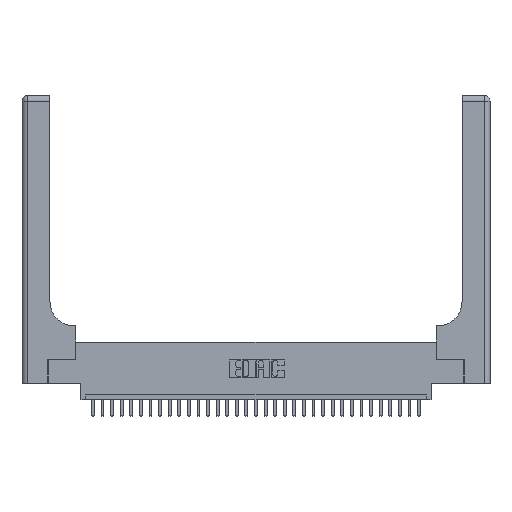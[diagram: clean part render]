
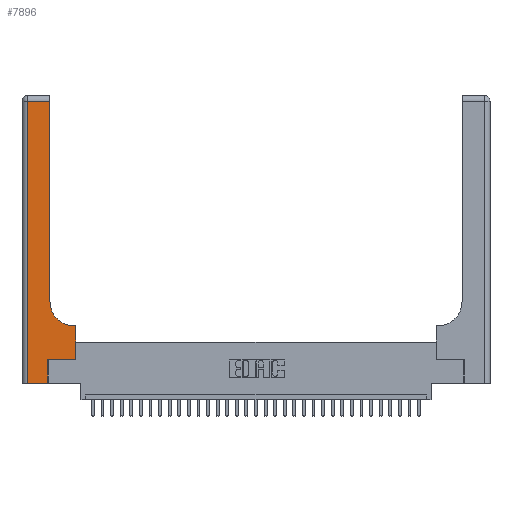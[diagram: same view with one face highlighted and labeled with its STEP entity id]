
A CAD part, top view. The second image highlights one B-rep face of the part: STEP entity #7896.
In plain terms, the highlighted planar face has unit normal (0, 0, 1).
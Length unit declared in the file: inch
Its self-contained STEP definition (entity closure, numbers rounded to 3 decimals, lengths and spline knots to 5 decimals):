
#596 = ORIENTED_EDGE ( 'NONE', *, *, #30596, .T. ) ;
#619 = LINE ( 'NONE', #20753, #26712 ) ;
#670 = VECTOR ( 'NONE', #19049, 39.37008 ) ;
#977 = ORIENTED_EDGE ( 'NONE', *, *, #3471, .T. ) ;
#1004 = VECTOR ( 'NONE', #30805, 39.37008 ) ;
#1244 = CARTESIAN_POINT ( 'NONE',  ( 0.5585, 0.25, 0.37 ) ) ;
#1308 = ORIENTED_EDGE ( 'NONE', *, *, #28252, .T. ) ;
#1707 = CARTESIAN_POINT ( 'NONE',  ( 0.2915, 2.94, 0.37 ) ) ;
#2346 = CARTESIAN_POINT ( 'NONE',  ( 0.5585, 0.6, 0.37 ) ) ;
#2643 = VERTEX_POINT ( 'NONE', #12329 ) ;
#2940 = VECTOR ( 'NONE', #27953, 39.37008 ) ;
#3414 = VERTEX_POINT ( 'NONE', #24376 ) ;
#3471 = EDGE_CURVE ( 'NONE', #3414, #27880, #11440, .T. ) ;
#3881 = CARTESIAN_POINT ( 'NONE',  ( 0.5585, 0.25, 0.37 ) ) ;
#4020 = CARTESIAN_POINT ( 'NONE',  ( 0.06, 3., 0.37 ) ) ;
#4110 = VERTEX_POINT ( 'NONE', #17464 ) ;
#4363 = AXIS2_PLACEMENT_3D ( 'NONE', #11455, #26843, #11352 ) ;
#4944 = CARTESIAN_POINT ( 'NONE',  ( 0., 2.94, 0.37 ) ) ;
#4988 = ORIENTED_EDGE ( 'NONE', *, *, #30149, .T. ) ;
#5148 = CARTESIAN_POINT ( 'NONE',  ( 0., 3., 0.37 ) ) ;
#5220 = CARTESIAN_POINT ( 'NONE',  ( 0.5415, 0.6, 0.37 ) ) ;
#5255 = EDGE_LOOP ( 'NONE', ( #6800, #1308, #977, #29255, #16577, #30570, #4988, #596, #31482 ) ) ;
#6446 = LINE ( 'NONE', #19573, #2940 ) ;
#6800 = ORIENTED_EDGE ( 'NONE', *, *, #17013, .T. ) ;
#7470 = DIRECTION ( 'NONE',  ( -1., 0., 0. ) ) ;
#7896 = ADVANCED_FACE ( 'NONE', ( #32536 ), #23077, .F. ) ;
#9350 = LINE ( 'NONE', #1244, #670 ) ;
#10486 = DIRECTION ( 'NONE',  ( 1., 0., 0. ) ) ;
#10885 = LINE ( 'NONE', #15597, #1004 ) ;
#11352 = DIRECTION ( 'NONE',  ( 1., 0., 0. ) ) ;
#11390 = VERTEX_POINT ( 'NONE', #1707 ) ;
#11440 = LINE ( 'NONE', #4020, #18214 ) ;
#11455 = CARTESIAN_POINT ( 'NONE',  ( 0.5415, 0.85, 0.37 ) ) ;
#11510 = DIRECTION ( 'NONE',  ( 0., -1., 0. ) ) ;
#12329 = CARTESIAN_POINT ( 'NONE',  ( 0.269, 0.25, 0.37 ) ) ;
#13341 = CARTESIAN_POINT ( 'NONE',  ( 0.06, 0., 0.37 ) ) ;
#13371 = LINE ( 'NONE', #28085, #31916 ) ;
#14637 = DIRECTION ( 'NONE',  ( 1., 0., 0. ) ) ;
#14687 = CARTESIAN_POINT ( 'NONE',  ( 0.269, 0., 0.37 ) ) ;
#15352 = VECTOR ( 'NONE', #14637, 39.37008 ) ;
#15490 = VERTEX_POINT ( 'NONE', #14687 ) ;
#15597 = CARTESIAN_POINT ( 'NONE',  ( 0.2915, 0.6, 0.37 ) ) ;
#16577 = ORIENTED_EDGE ( 'NONE', *, *, #17888, .T. ) ;
#17013 = EDGE_CURVE ( 'NONE', #4110, #11390, #619, .T. ) ;
#17464 = CARTESIAN_POINT ( 'NONE',  ( 0.2915, 0.85, 0.37 ) ) ;
#17708 = LINE ( 'NONE', #19840, #15352 ) ;
#17888 = EDGE_CURVE ( 'NONE', #15490, #2643, #6446, .T. ) ;
#18214 = VECTOR ( 'NONE', #11510, 39.37008 ) ;
#18668 = EDGE_CURVE ( 'NONE', #27880, #15490, #13371, .T. ) ;
#19049 = DIRECTION ( 'NONE',  ( 0., 1., 0. ) ) ;
#19573 = CARTESIAN_POINT ( 'NONE',  ( 0.269, 0., 0.37 ) ) ;
#19840 = CARTESIAN_POINT ( 'NONE',  ( 0.269, 0.25, 0.37 ) ) ;
#20753 = CARTESIAN_POINT ( 'NONE',  ( 0.2915, 3., 0.37 ) ) ;
#22767 = DIRECTION ( 'NONE',  ( -1., 0., 0. ) ) ;
#23077 = PLANE ( 'NONE',  #29930 ) ;
#23827 = DIRECTION ( 'NONE',  ( 0., 1., 0. ) ) ;
#23837 = VECTOR ( 'NONE', #7470, 39.37008 ) ;
#23954 = VERTEX_POINT ( 'NONE', #5220 ) ;
#24376 = CARTESIAN_POINT ( 'NONE',  ( 0.06, 2.94, 0.37 ) ) ;
#26712 = VECTOR ( 'NONE', #23827, 39.37008 ) ;
#26843 = DIRECTION ( 'NONE',  ( 0., 0., -1. ) ) ;
#26943 = EDGE_CURVE ( 'NONE', #2643, #27402, #17708, .T. ) ;
#27402 = VERTEX_POINT ( 'NONE', #3881 ) ;
#27695 = VERTEX_POINT ( 'NONE', #2346 ) ;
#27880 = VERTEX_POINT ( 'NONE', #13341 ) ;
#27919 = DIRECTION ( 'NONE',  ( 0., 0., -1. ) ) ;
#27953 = DIRECTION ( 'NONE',  ( 0., 1., 0. ) ) ;
#28085 = CARTESIAN_POINT ( 'NONE',  ( 0., 0., 0.37 ) ) ;
#28252 = EDGE_CURVE ( 'NONE', #11390, #3414, #30910, .T. ) ;
#29255 = ORIENTED_EDGE ( 'NONE', *, *, #18668, .T. ) ;
#29930 = AXIS2_PLACEMENT_3D ( 'NONE', #5148, #27919, #22767 ) ;
#30149 = EDGE_CURVE ( 'NONE', #27402, #27695, #9350, .T. ) ;
#30216 = CIRCLE ( 'NONE', #4363, 0.25 ) ;
#30570 = ORIENTED_EDGE ( 'NONE', *, *, #26943, .T. ) ;
#30596 = EDGE_CURVE ( 'NONE', #27695, #23954, #10885, .T. ) ;
#30783 = EDGE_CURVE ( 'NONE', #23954, #4110, #30216, .T. ) ;
#30805 = DIRECTION ( 'NONE',  ( -1., 0., 0. ) ) ;
#30910 = LINE ( 'NONE', #4944, #23837 ) ;
#31482 = ORIENTED_EDGE ( 'NONE', *, *, #30783, .T. ) ;
#31916 = VECTOR ( 'NONE', #10486, 39.37008 ) ;
#32536 = FACE_OUTER_BOUND ( 'NONE', #5255, .T. ) ;
